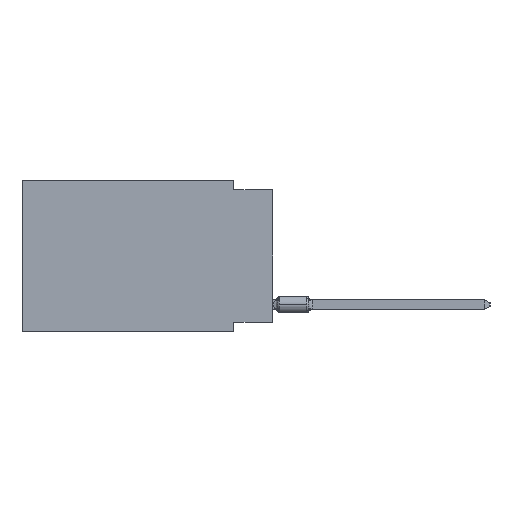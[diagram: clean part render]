
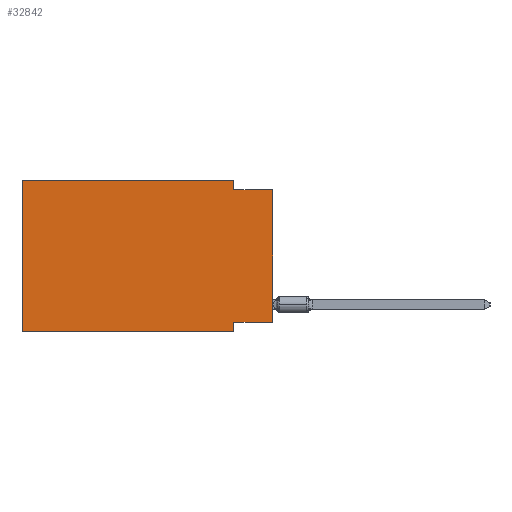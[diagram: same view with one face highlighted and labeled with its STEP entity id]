
A CAD part, left-side view. The second image highlights one B-rep face of the part: STEP entity #32842.
In plain terms, the highlighted planar face has unit normal (-1, 0, 0).
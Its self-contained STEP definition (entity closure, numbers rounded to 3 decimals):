
#1417 = ORIENTED_EDGE ( 'NONE', *, *, #28039, .F. ) ;
#3099 = AXIS2_PLACEMENT_3D ( 'NONE', #37037, #28963, #6189 ) ;
#3114 = ORIENTED_EDGE ( 'NONE', *, *, #39776, .F. ) ;
#6149 = CARTESIAN_POINT ( 'NONE',  ( 0., 2.54, 0. ) ) ;
#6189 = DIRECTION ( 'NONE',  ( 0., 0., -1. ) ) ;
#6374 = DIRECTION ( 'NONE',  ( 0., -1., 0. ) ) ;
#7253 = EDGE_CURVE ( 'NONE', #35372, #17406, #47596, .T. ) ;
#7457 = CARTESIAN_POINT ( 'NONE',  ( 0., 0., -9.271 ) ) ;
#9717 = LINE ( 'NONE', #13162, #17152 ) ;
#10550 = DIRECTION ( 'NONE',  ( 0., 0., -1. ) ) ;
#10585 = PLANE ( 'NONE',  #3099 ) ;
#11468 = EDGE_CURVE ( 'NONE', #12427, #12125, #38715, .T. ) ;
#12125 = VERTEX_POINT ( 'NONE', #24478 ) ;
#12427 = VERTEX_POINT ( 'NONE', #31226 ) ;
#13162 = CARTESIAN_POINT ( 'NONE',  ( 0., 0., 0. ) ) ;
#13270 = LINE ( 'NONE', #6149, #38106 ) ;
#13589 = DIRECTION ( 'NONE',  ( 0., 0., 1. ) ) ;
#13746 = CARTESIAN_POINT ( 'NONE',  ( 0., 16.383, 0. ) ) ;
#15543 = DIRECTION ( 'NONE',  ( 0., -1., 0. ) ) ;
#17152 = VECTOR ( 'NONE', #24414, 1000. ) ;
#17406 = VERTEX_POINT ( 'NONE', #13746 ) ;
#18160 = VECTOR ( 'NONE', #23302, 1000. ) ;
#19132 = EDGE_LOOP ( 'NONE', ( #38531, #47465, #1417, #3114, #43169, #19861, #45321, #31973 ) ) ;
#19861 = ORIENTED_EDGE ( 'NONE', *, *, #21535, .T. ) ;
#21095 = LINE ( 'NONE', #42644, #28599 ) ;
#21535 = EDGE_CURVE ( 'NONE', #35372, #12125, #23105, .T. ) ;
#22505 = EDGE_CURVE ( 'NONE', #26302, #12427, #43041, .T. ) ;
#23070 = CARTESIAN_POINT ( 'NONE',  ( 0., 2.54, -9.906 ) ) ;
#23105 = LINE ( 'NONE', #30929, #31429 ) ;
#23302 = DIRECTION ( 'NONE',  ( 0., 0., -1. ) ) ;
#23614 = VECTOR ( 'NONE', #13589, 1000. ) ;
#24414 = DIRECTION ( 'NONE',  ( 0., 0., 1. ) ) ;
#24478 = CARTESIAN_POINT ( 'NONE',  ( 0., 2.54, -9.906 ) ) ;
#24901 = DIRECTION ( 'NONE',  ( 0., 1., 0. ) ) ;
#25200 = CARTESIAN_POINT ( 'NONE',  ( 0., 16.383, -9.906 ) ) ;
#26302 = VERTEX_POINT ( 'NONE', #7457 ) ;
#26616 = CARTESIAN_POINT ( 'NONE',  ( 0., 2.54, -0.635 ) ) ;
#28039 = EDGE_CURVE ( 'NONE', #47152, #43459, #13270, .T. ) ;
#28347 = CARTESIAN_POINT ( 'NONE',  ( 0., 0., -9.271 ) ) ;
#28599 = VECTOR ( 'NONE', #31140, 1000. ) ;
#28963 = DIRECTION ( 'NONE',  ( 1., 0., 0. ) ) ;
#29009 = VECTOR ( 'NONE', #6374, 1000. ) ;
#30929 = CARTESIAN_POINT ( 'NONE',  ( 0., 16.383, -9.906 ) ) ;
#31140 = DIRECTION ( 'NONE',  ( 0., -1., 0. ) ) ;
#31226 = CARTESIAN_POINT ( 'NONE',  ( 0., 2.54, -9.271 ) ) ;
#31429 = VECTOR ( 'NONE', #15543, 1000. ) ;
#31973 = ORIENTED_EDGE ( 'NONE', *, *, #22505, .F. ) ;
#32150 = FACE_OUTER_BOUND ( 'NONE', #19132, .T. ) ;
#32189 = CARTESIAN_POINT ( 'NONE',  ( 0., 16.383, 0. ) ) ;
#32587 = CARTESIAN_POINT ( 'NONE',  ( 0., 16.383, 0. ) ) ;
#32842 = ADVANCED_FACE ( 'NONE', ( #32150 ), #10585, .F. ) ;
#35372 = VERTEX_POINT ( 'NONE', #25200 ) ;
#35714 = EDGE_CURVE ( 'NONE', #26302, #39336, #9717, .T. ) ;
#37037 = CARTESIAN_POINT ( 'NONE',  ( 0., 16.383, 0. ) ) ;
#38106 = VECTOR ( 'NONE', #10550, 1000. ) ;
#38531 = ORIENTED_EDGE ( 'NONE', *, *, #35714, .T. ) ;
#38715 = LINE ( 'NONE', #23070, #18160 ) ;
#39336 = VERTEX_POINT ( 'NONE', #43676 ) ;
#39776 = EDGE_CURVE ( 'NONE', #17406, #47152, #47273, .T. ) ;
#41985 = CARTESIAN_POINT ( 'NONE',  ( 0., 2.54, 0. ) ) ;
#42644 = CARTESIAN_POINT ( 'NONE',  ( 0., 0., -0.635 ) ) ;
#43041 = LINE ( 'NONE', #28347, #46268 ) ;
#43169 = ORIENTED_EDGE ( 'NONE', *, *, #7253, .F. ) ;
#43459 = VERTEX_POINT ( 'NONE', #26616 ) ;
#43676 = CARTESIAN_POINT ( 'NONE',  ( 0., 0., -0.635 ) ) ;
#45321 = ORIENTED_EDGE ( 'NONE', *, *, #11468, .F. ) ;
#45608 = EDGE_CURVE ( 'NONE', #43459, #39336, #21095, .T. ) ;
#46268 = VECTOR ( 'NONE', #24901, 1000. ) ;
#47152 = VERTEX_POINT ( 'NONE', #41985 ) ;
#47273 = LINE ( 'NONE', #32587, #29009 ) ;
#47465 = ORIENTED_EDGE ( 'NONE', *, *, #45608, .F. ) ;
#47596 = LINE ( 'NONE', #32189, #23614 ) ;
